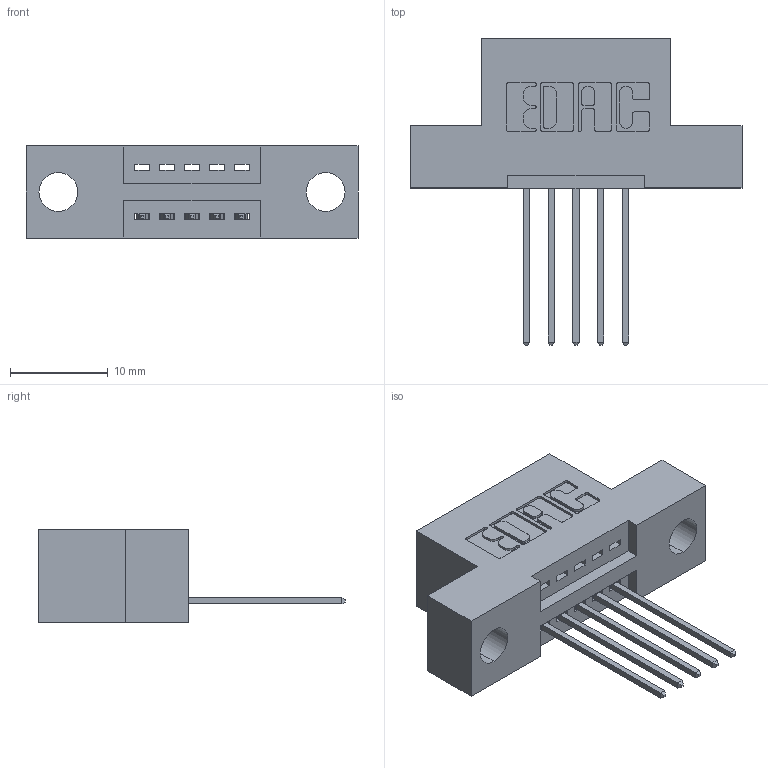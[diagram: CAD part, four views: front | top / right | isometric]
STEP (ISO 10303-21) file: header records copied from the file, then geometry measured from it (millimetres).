
FILE_DESCRIPTION (( 'STEP AP203' ), '1' );
FILE_NAME ('345-005-542-104.STEP', '2021-05-26T13:58:53', ( '' ), ( '' ), 'SwSTEP 2.0', 'SolidWorks 2020', '' );
FILE_SCHEMA (( 'CONFIG_CONTROL_DESIGN' ));
Length unit declared in the file: inch
Products named in the file (3): 345-005-542-104; 345 Part_Flush Mounting Lugs - 0.156 Dia-TI; 345-292-001_345-293-142
Assembly tree (6 placements, depth 2):
  345-005-542-104
    345 Part_Flush Mounting Lugs - 0.156 Dia-TI
    345-292-001_345-293-142  x5
Bounding box: 33.91 x 31.29 x 9.4 mm (x, y, z)
Volume: 2822.8 mm3; surface area: 3161.2 mm2
Topology: 6 solids, 6 shells, 430 faces, 1257 edges, 830 vertices
Faces by surface type: plane 294, cylinder 136
Entity records: 9181 total; most frequent: CARTESIAN_POINT 1601, ORIENTED_EDGE 1538, DIRECTION 1451, EDGE_CURVE 769, LINE 617, VECTOR 617, VERTEX_POINT 510, AXIS2_PLACEMENT_3D 417
